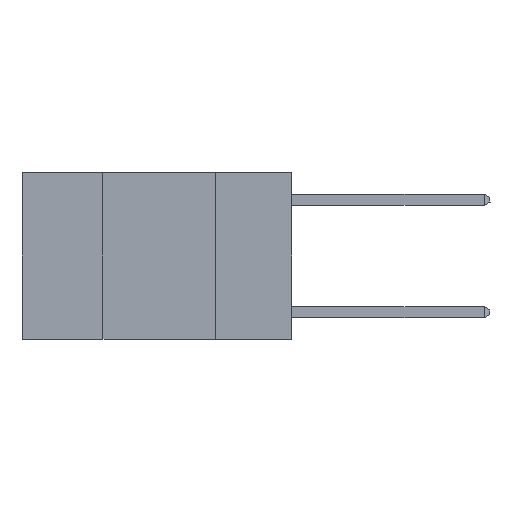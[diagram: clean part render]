
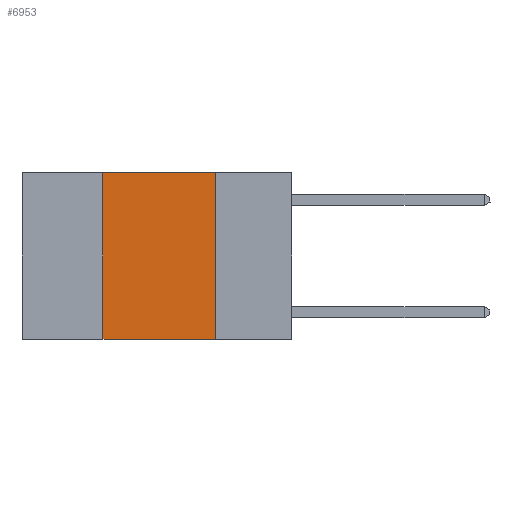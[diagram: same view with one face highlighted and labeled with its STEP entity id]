
A CAD part, left-side view. The second image highlights one B-rep face of the part: STEP entity #6953.
In plain terms, the highlighted planar face has unit normal (-1, 0, 0).
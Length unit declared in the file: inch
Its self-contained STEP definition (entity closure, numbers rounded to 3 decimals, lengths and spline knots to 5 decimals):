
#1821 = VERTEX_POINT ( 'NONE', #10219 ) ;
#2430 = VECTOR ( 'NONE', #6170, 39.37008 ) ;
#2506 = CARTESIAN_POINT ( 'NONE',  ( 0., 0.42, -0.37 ) ) ;
#2657 = VERTEX_POINT ( 'NONE', #2506 ) ;
#2721 = DIRECTION ( 'NONE',  ( 1., 0., 0. ) ) ;
#2834 = VERTEX_POINT ( 'NONE', #2910 ) ;
#2910 = CARTESIAN_POINT ( 'NONE',  ( 0., 0.42, 0. ) ) ;
#3484 = VERTEX_POINT ( 'NONE', #7289 ) ;
#3818 = EDGE_LOOP ( 'NONE', ( #9128, #7019, #7295, #5241 ) ) ;
#4383 = EDGE_CURVE ( 'NONE', #3484, #1821, #8445, .T. ) ;
#4425 = VECTOR ( 'NONE', #4543, 39.37008 ) ;
#4514 = CARTESIAN_POINT ( 'NONE',  ( 0., 0.6, 0. ) ) ;
#4543 = DIRECTION ( 'NONE',  ( 0., 0., 1. ) ) ;
#5199 = EDGE_CURVE ( 'NONE', #2657, #1821, #9819, .T. ) ;
#5241 = ORIENTED_EDGE ( 'NONE', *, *, #5199, .T. ) ;
#5330 = VECTOR ( 'NONE', #11541, 39.37008 ) ;
#5384 = VECTOR ( 'NONE', #10812, 39.37008 ) ;
#5481 = CARTESIAN_POINT ( 'NONE',  ( 0., 0.6, -0.37 ) ) ;
#6170 = DIRECTION ( 'NONE',  ( 0., 0., -1. ) ) ;
#6527 = AXIS2_PLACEMENT_3D ( 'NONE', #4514, #2721, #8982 ) ;
#6953 = ADVANCED_FACE ( 'NONE', ( #8525 ), #8067, .F. ) ;
#7019 = ORIENTED_EDGE ( 'NONE', *, *, #7435, .F. ) ;
#7289 = CARTESIAN_POINT ( 'NONE',  ( 0., 0.17, 0. ) ) ;
#7295 = ORIENTED_EDGE ( 'NONE', *, *, #8760, .F. ) ;
#7435 = EDGE_CURVE ( 'NONE', #2834, #3484, #8225, .T. ) ;
#7588 = LINE ( 'NONE', #8967, #4425 ) ;
#8067 = PLANE ( 'NONE',  #6527 ) ;
#8225 = LINE ( 'NONE', #8823, #5330 ) ;
#8445 = LINE ( 'NONE', #9678, #2430 ) ;
#8525 = FACE_OUTER_BOUND ( 'NONE', #3818, .T. ) ;
#8760 = EDGE_CURVE ( 'NONE', #2657, #2834, #7588, .T. ) ;
#8823 = CARTESIAN_POINT ( 'NONE',  ( 0., 0.6, 0. ) ) ;
#8967 = CARTESIAN_POINT ( 'NONE',  ( 0., 0.42, 0. ) ) ;
#8982 = DIRECTION ( 'NONE',  ( 0., 0., -1. ) ) ;
#9128 = ORIENTED_EDGE ( 'NONE', *, *, #4383, .F. ) ;
#9678 = CARTESIAN_POINT ( 'NONE',  ( 0., 0.17, 0. ) ) ;
#9819 = LINE ( 'NONE', #5481, #5384 ) ;
#10219 = CARTESIAN_POINT ( 'NONE',  ( 0., 0.17, -0.37 ) ) ;
#10812 = DIRECTION ( 'NONE',  ( 0., -1., 0. ) ) ;
#11541 = DIRECTION ( 'NONE',  ( 0., -1., 0. ) ) ;
